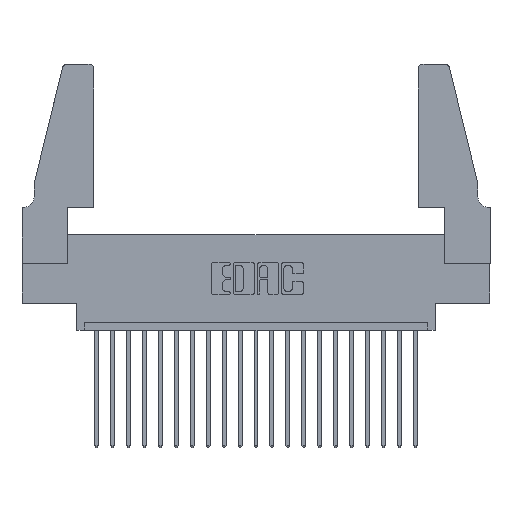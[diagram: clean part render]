
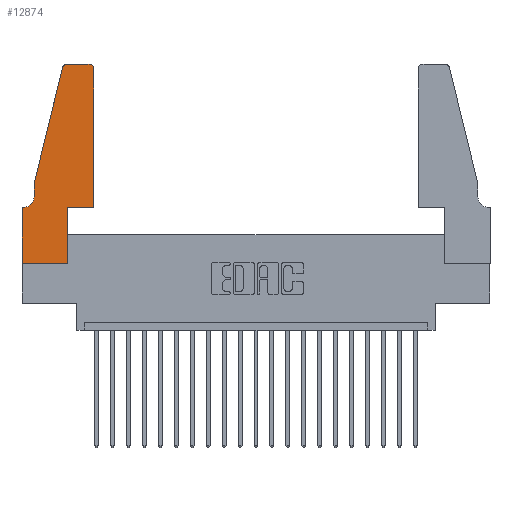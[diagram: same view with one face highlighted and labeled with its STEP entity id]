
A CAD part, top view. The second image highlights one B-rep face of the part: STEP entity #12874.
In plain terms, the highlighted planar face has unit normal (0, 0, 1).
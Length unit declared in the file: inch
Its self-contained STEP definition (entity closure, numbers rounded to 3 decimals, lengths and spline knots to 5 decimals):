
#68 = VERTEX_POINT ( 'NONE', #5966 ) ;
#247 = CARTESIAN_POINT ( 'NONE',  ( 0., 0.35, 0.37 ) ) ;
#267 = CARTESIAN_POINT ( 'NONE',  ( 0., 0., 0.37 ) ) ;
#274 = VECTOR ( 'NONE', #1900, 39.37008 ) ;
#429 = EDGE_CURVE ( 'NONE', #2823, #2994, #18380, .T. ) ;
#913 = ORIENTED_EDGE ( 'NONE', *, *, #4148, .T. ) ;
#1155 = AXIS2_PLACEMENT_3D ( 'NONE', #247, #13421, #2183 ) ;
#1158 = CARTESIAN_POINT ( 'NONE',  ( 0.2865, 0.35, 0.37 ) ) ;
#1574 = VECTOR ( 'NONE', #14805, 39.37008 ) ;
#1688 = LINE ( 'NONE', #17961, #16877 ) ;
#1852 = CARTESIAN_POINT ( 'NONE',  ( 0., 0., 0.37 ) ) ;
#1900 = DIRECTION ( 'NONE',  ( -1., 0., 0. ) ) ;
#2073 = AXIS2_PLACEMENT_3D ( 'NONE', #15116, #18381, #7148 ) ;
#2183 = DIRECTION ( 'NONE',  ( 1., 0., 0. ) ) ;
#2291 = CARTESIAN_POINT ( 'NONE',  ( 0., 0.35, 0.37 ) ) ;
#2379 = VERTEX_POINT ( 'NONE', #17357 ) ;
#2506 = DIRECTION ( 'NONE',  ( 0., 1., 0. ) ) ;
#2725 = VECTOR ( 'NONE', #16751, 39.37008 ) ;
#2823 = VERTEX_POINT ( 'NONE', #17022 ) ;
#2994 = VERTEX_POINT ( 'NONE', #14620 ) ;
#2997 = VECTOR ( 'NONE', #17324, 39.37008 ) ;
#3009 = VERTEX_POINT ( 'NONE', #14417 ) ;
#3262 = ORIENTED_EDGE ( 'NONE', *, *, #13971, .T. ) ;
#3285 = EDGE_CURVE ( 'NONE', #68, #2823, #8913, .T. ) ;
#3380 = VERTEX_POINT ( 'NONE', #14675 ) ;
#3869 = ORIENTED_EDGE ( 'NONE', *, *, #7807, .T. ) ;
#3924 = DIRECTION ( 'NONE',  ( 0., 1., 0. ) ) ;
#4004 = DIRECTION ( 'NONE',  ( 0., 0., 1. ) ) ;
#4148 = EDGE_CURVE ( 'NONE', #20729, #3380, #11123, .T. ) ;
#5032 = VECTOR ( 'NONE', #10331, 39.37008 ) ;
#5046 = ORIENTED_EDGE ( 'NONE', *, *, #11860, .T. ) ;
#5186 = EDGE_CURVE ( 'NONE', #11415, #2379, #6812, .T. ) ;
#5242 = PLANE ( 'NONE',  #1155 ) ;
#5287 = AXIS2_PLACEMENT_3D ( 'NONE', #15141, #4004, #8738 ) ;
#5452 = CARTESIAN_POINT ( 'NONE',  ( 0.284, 1.22, 0.37 ) ) ;
#5676 = LINE ( 'NONE', #18070, #1574 ) ;
#5966 = CARTESIAN_POINT ( 'NONE',  ( 0.4205, 1.25, 0.37 ) ) ;
#6557 = LINE ( 'NONE', #1852, #7321 ) ;
#6663 = ORIENTED_EDGE ( 'NONE', *, *, #7023, .T. ) ;
#6812 = LINE ( 'NONE', #9146, #2997 ) ;
#6939 = CARTESIAN_POINT ( 'NONE',  ( 0., 0., 0.37 ) ) ;
#6946 = VERTEX_POINT ( 'NONE', #2291 ) ;
#7023 = EDGE_CURVE ( 'NONE', #6946, #16289, #6557, .T. ) ;
#7148 = DIRECTION ( 'NONE',  ( -1., 0., 0. ) ) ;
#7321 = VECTOR ( 'NONE', #11535, 39.37008 ) ;
#7807 = EDGE_CURVE ( 'NONE', #3380, #68, #17624, .T. ) ;
#8346 = CARTESIAN_POINT ( 'NONE',  ( 0.2605, 1.25, 0.37 ) ) ;
#8738 = DIRECTION ( 'NONE',  ( 1., 0., 0. ) ) ;
#8913 = LINE ( 'NONE', #8346, #274 ) ;
#9146 = CARTESIAN_POINT ( 'NONE',  ( 0.0755, 0.5, 0.37 ) ) ;
#10086 = LINE ( 'NONE', #6939, #5032 ) ;
#10148 = VECTOR ( 'NONE', #2506, 39.37008 ) ;
#10331 = DIRECTION ( 'NONE',  ( 1., 0., 0. ) ) ;
#10383 = VERTEX_POINT ( 'NONE', #14645 ) ;
#10564 = ORIENTED_EDGE ( 'NONE', *, *, #429, .T. ) ;
#10570 = LINE ( 'NONE', #18395, #2725 ) ;
#11123 = LINE ( 'NONE', #20028, #10148 ) ;
#11415 = VERTEX_POINT ( 'NONE', #18552 ) ;
#11535 = DIRECTION ( 'NONE',  ( 0., -1., 0. ) ) ;
#11830 = EDGE_CURVE ( 'NONE', #10383, #16061, #1688, .T. ) ;
#11860 = EDGE_CURVE ( 'NONE', #2994, #11415, #10570, .T. ) ;
#12268 = FACE_OUTER_BOUND ( 'NONE', #13056, .T. ) ;
#12706 = EDGE_CURVE ( 'NONE', #2379, #3009, #16835, .T. ) ;
#12874 = ADVANCED_FACE ( 'NONE', ( #12268 ), #5242, .T. ) ;
#13056 = EDGE_LOOP ( 'NONE', ( #16490, #10564, #5046, #19421, #13372, #3262, #6663, #19893, #17580, #17398, #913, #3869 ) ) ;
#13372 = ORIENTED_EDGE ( 'NONE', *, *, #12706, .T. ) ;
#13421 = DIRECTION ( 'NONE',  ( 0., 0., 1. ) ) ;
#13541 = VECTOR ( 'NONE', #15851, 39.37008 ) ;
#13971 = EDGE_CURVE ( 'NONE', #3009, #6946, #17553, .T. ) ;
#14417 = CARTESIAN_POINT ( 'NONE',  ( 0.0055, 0.35, 0.37 ) ) ;
#14620 = CARTESIAN_POINT ( 'NONE',  ( 0.25487, 1.22718, 0.37 ) ) ;
#14645 = CARTESIAN_POINT ( 'NONE',  ( 0.2865, 0., 0.37 ) ) ;
#14675 = CARTESIAN_POINT ( 'NONE',  ( 0.4505, 1.22, 0.37 ) ) ;
#14805 = DIRECTION ( 'NONE',  ( 1., 0., 0. ) ) ;
#15092 = EDGE_CURVE ( 'NONE', #16061, #20729, #5676, .T. ) ;
#15116 = CARTESIAN_POINT ( 'NONE',  ( 0.0055, 0.42, 0.37 ) ) ;
#15141 = CARTESIAN_POINT ( 'NONE',  ( 0.4205, 1.22, 0.37 ) ) ;
#15851 = DIRECTION ( 'NONE',  ( -1., 0., 0. ) ) ;
#16061 = VERTEX_POINT ( 'NONE', #1158 ) ;
#16289 = VERTEX_POINT ( 'NONE', #267 ) ;
#16490 = ORIENTED_EDGE ( 'NONE', *, *, #3285, .T. ) ;
#16751 = DIRECTION ( 'NONE',  ( -0.239, -0.971, 0. ) ) ;
#16835 = CIRCLE ( 'NONE', #2073, 0.07 ) ;
#16877 = VECTOR ( 'NONE', #3924, 39.37008 ) ;
#17022 = CARTESIAN_POINT ( 'NONE',  ( 0.284, 1.25, 0.37 ) ) ;
#17324 = DIRECTION ( 'NONE',  ( 0., -1., 0. ) ) ;
#17357 = CARTESIAN_POINT ( 'NONE',  ( 0.0755, 0.42, 0.37 ) ) ;
#17398 = ORIENTED_EDGE ( 'NONE', *, *, #15092, .T. ) ;
#17510 = EDGE_CURVE ( 'NONE', #16289, #10383, #10086, .T. ) ;
#17553 = LINE ( 'NONE', #19183, #13541 ) ;
#17580 = ORIENTED_EDGE ( 'NONE', *, *, #11830, .T. ) ;
#17624 = CIRCLE ( 'NONE', #5287, 0.03 ) ;
#17671 = CARTESIAN_POINT ( 'NONE',  ( 0.4505, 0.35, 0.37 ) ) ;
#17961 = CARTESIAN_POINT ( 'NONE',  ( 0.2865, 0.35, 0.37 ) ) ;
#18070 = CARTESIAN_POINT ( 'NONE',  ( 0.4505, 0.35, 0.37 ) ) ;
#18380 = CIRCLE ( 'NONE', #18469, 0.03 ) ;
#18381 = DIRECTION ( 'NONE',  ( 0., 0., -1. ) ) ;
#18395 = CARTESIAN_POINT ( 'NONE',  ( 0.0755, 0.5, 0.37 ) ) ;
#18431 = DIRECTION ( 'NONE',  ( 1., 0., 0. ) ) ;
#18469 = AXIS2_PLACEMENT_3D ( 'NONE', #5452, #19915, #18431 ) ;
#18552 = CARTESIAN_POINT ( 'NONE',  ( 0.0755, 0.5, 0.37 ) ) ;
#19183 = CARTESIAN_POINT ( 'NONE',  ( 0.0755, 0.35, 0.37 ) ) ;
#19421 = ORIENTED_EDGE ( 'NONE', *, *, #5186, .T. ) ;
#19893 = ORIENTED_EDGE ( 'NONE', *, *, #17510, .T. ) ;
#19915 = DIRECTION ( 'NONE',  ( 0., 0., 1. ) ) ;
#20028 = CARTESIAN_POINT ( 'NONE',  ( 0.4505, 0.35, 0.37 ) ) ;
#20729 = VERTEX_POINT ( 'NONE', #17671 ) ;
